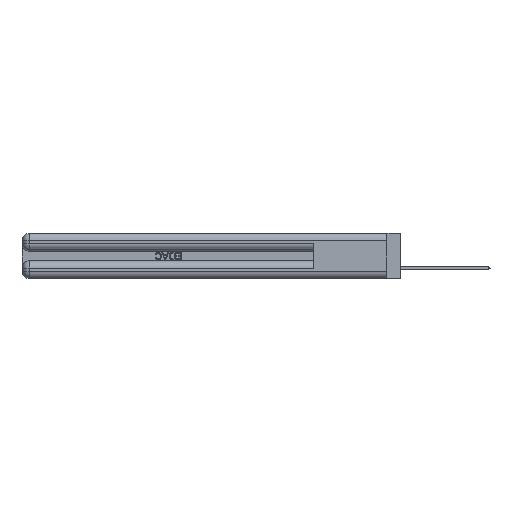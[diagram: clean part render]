
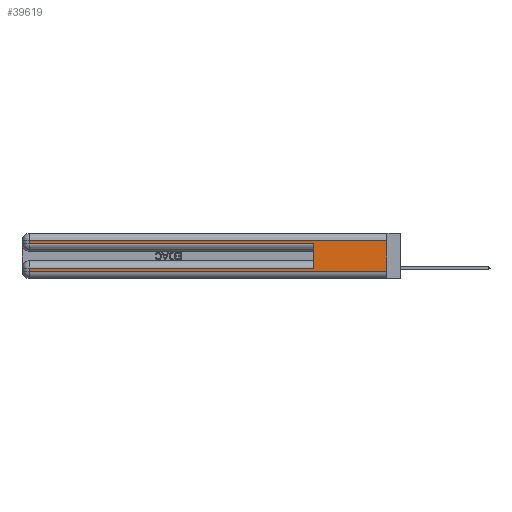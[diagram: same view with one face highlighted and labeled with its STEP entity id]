
A CAD part, left-side view. The second image highlights one B-rep face of the part: STEP entity #39619.
In plain terms, the highlighted planar face has unit normal (-1, 0, 0).
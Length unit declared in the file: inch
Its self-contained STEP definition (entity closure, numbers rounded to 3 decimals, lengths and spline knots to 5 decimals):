
#538 = ORIENTED_EDGE ( 'NONE', *, *, #32145, .F. ) ;
#1326 = DIRECTION ( 'NONE',  ( 0., 0., -1. ) ) ;
#2023 = EDGE_CURVE ( 'NONE', #17741, #42059, #13744, .T. ) ;
#2118 = EDGE_CURVE ( 'NONE', #23385, #24872, #3670, .T. ) ;
#2363 = CARTESIAN_POINT ( 'NONE',  ( 0., 0.6, 0.085 ) ) ;
#2894 = DIRECTION ( 'NONE',  ( 0., 1., 0. ) ) ;
#3670 = LINE ( 'NONE', #36742, #14891 ) ;
#6598 = CARTESIAN_POINT ( 'NONE',  ( 0., 2.94, 0.285 ) ) ;
#7458 = VECTOR ( 'NONE', #41782, 39.37008 ) ;
#7958 = CARTESIAN_POINT ( 'NONE',  ( 0., 2.94, 0.06 ) ) ;
#8704 = EDGE_CURVE ( 'NONE', #26490, #17741, #18609, .T. ) ;
#8766 = VERTEX_POINT ( 'NONE', #2363 ) ;
#8827 = LINE ( 'NONE', #45087, #42312 ) ;
#8953 = CARTESIAN_POINT ( 'NONE',  ( 0., 2.94, 0.31 ) ) ;
#9788 = ORIENTED_EDGE ( 'NONE', *, *, #39376, .T. ) ;
#10884 = ORIENTED_EDGE ( 'NONE', *, *, #35740, .T. ) ;
#11084 = ORIENTED_EDGE ( 'NONE', *, *, #2023, .T. ) ;
#11558 = ORIENTED_EDGE ( 'NONE', *, *, #2118, .T. ) ;
#12390 = VECTOR ( 'NONE', #2894, 39.37008 ) ;
#13744 = LINE ( 'NONE', #25308, #23661 ) ;
#13808 = EDGE_CURVE ( 'NONE', #23385, #42059, #24489, .T. ) ;
#13903 = PLANE ( 'NONE',  #44922 ) ;
#13957 = VERTEX_POINT ( 'NONE', #6598 ) ;
#14132 = VECTOR ( 'NONE', #32465, 39.37008 ) ;
#14891 = VECTOR ( 'NONE', #28653, 39.37008 ) ;
#15364 = CARTESIAN_POINT ( 'NONE',  ( 0., 0.6, 0.145 ) ) ;
#16976 = CARTESIAN_POINT ( 'NONE',  ( 0., 2.94, 0.37 ) ) ;
#17634 = DIRECTION ( 'NONE',  ( 0., 0., -1. ) ) ;
#17741 = VERTEX_POINT ( 'NONE', #7958 ) ;
#17800 = CARTESIAN_POINT ( 'NONE',  ( 0., 0., 0.37 ) ) ;
#18609 = LINE ( 'NONE', #35042, #19756 ) ;
#19756 = VECTOR ( 'NONE', #1326, 39.37008 ) ;
#22577 = DIRECTION ( 'NONE',  ( 0., -1., 0. ) ) ;
#23291 = LINE ( 'NONE', #15364, #7458 ) ;
#23385 = VERTEX_POINT ( 'NONE', #24421 ) ;
#23661 = VECTOR ( 'NONE', #36323, 39.37008 ) ;
#24160 = ORIENTED_EDGE ( 'NONE', *, *, #13808, .F. ) ;
#24421 = CARTESIAN_POINT ( 'NONE',  ( 0., 0., 0.31 ) ) ;
#24489 = LINE ( 'NONE', #17800, #33348 ) ;
#24872 = VERTEX_POINT ( 'NONE', #8953 ) ;
#25117 = CARTESIAN_POINT ( 'NONE',  ( 0., 0., 0.06 ) ) ;
#25308 = CARTESIAN_POINT ( 'NONE',  ( 0., 0., 0.06 ) ) ;
#26490 = VERTEX_POINT ( 'NONE', #48498 ) ;
#28653 = DIRECTION ( 'NONE',  ( 0., 1., 0. ) ) ;
#31727 = LINE ( 'NONE', #16976, #14132 ) ;
#32145 = EDGE_CURVE ( 'NONE', #8766, #45036, #23291, .T. ) ;
#32465 = DIRECTION ( 'NONE',  ( 0., 0., -1. ) ) ;
#33348 = VECTOR ( 'NONE', #44103, 39.37008 ) ;
#33458 = CARTESIAN_POINT ( 'NONE',  ( 0., 0., 0.085 ) ) ;
#34193 = LINE ( 'NONE', #33458, #12390 ) ;
#34564 = ORIENTED_EDGE ( 'NONE', *, *, #8704, .T. ) ;
#34620 = FACE_OUTER_BOUND ( 'NONE', #38902, .T. ) ;
#35026 = CARTESIAN_POINT ( 'NONE',  ( 0., 0.6, 0.285 ) ) ;
#35042 = CARTESIAN_POINT ( 'NONE',  ( 0., 2.94, 0.37 ) ) ;
#35740 = EDGE_CURVE ( 'NONE', #8766, #26490, #34193, .T. ) ;
#36323 = DIRECTION ( 'NONE',  ( 0., -1., 0. ) ) ;
#36742 = CARTESIAN_POINT ( 'NONE',  ( 0., 0., 0.31 ) ) ;
#38433 = EDGE_CURVE ( 'NONE', #13957, #45036, #8827, .T. ) ;
#38902 = EDGE_LOOP ( 'NONE', ( #24160, #11558, #9788, #44433, #538, #10884, #34564, #11084 ) ) ;
#39376 = EDGE_CURVE ( 'NONE', #24872, #13957, #31727, .T. ) ;
#39619 = ADVANCED_FACE ( 'NONE', ( #34620 ), #13903, .F. ) ;
#40171 = DIRECTION ( 'NONE',  ( 1., 0., 0. ) ) ;
#40497 = CARTESIAN_POINT ( 'NONE',  ( 0., 0., 0.37 ) ) ;
#41782 = DIRECTION ( 'NONE',  ( 0., 0., 1. ) ) ;
#42059 = VERTEX_POINT ( 'NONE', #25117 ) ;
#42312 = VECTOR ( 'NONE', #22577, 39.37008 ) ;
#44103 = DIRECTION ( 'NONE',  ( 0., 0., -1. ) ) ;
#44433 = ORIENTED_EDGE ( 'NONE', *, *, #38433, .T. ) ;
#44922 = AXIS2_PLACEMENT_3D ( 'NONE', #40497, #40171, #17634 ) ;
#45036 = VERTEX_POINT ( 'NONE', #35026 ) ;
#45087 = CARTESIAN_POINT ( 'NONE',  ( 0., 0., 0.285 ) ) ;
#48498 = CARTESIAN_POINT ( 'NONE',  ( 0., 2.94, 0.085 ) ) ;
